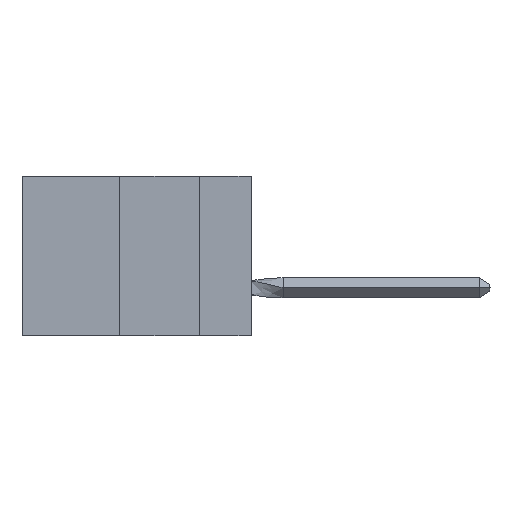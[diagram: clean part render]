
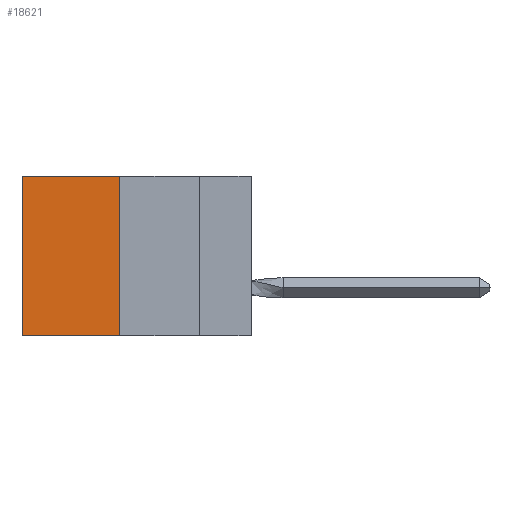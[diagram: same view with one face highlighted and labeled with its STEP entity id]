
A CAD part, left-side view. The second image highlights one B-rep face of the part: STEP entity #18621.
In plain terms, the highlighted planar face has unit normal (-1, 0, 0).
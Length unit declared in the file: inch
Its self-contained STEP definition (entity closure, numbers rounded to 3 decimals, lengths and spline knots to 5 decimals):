
#659 = CARTESIAN_POINT ( 'NONE',  ( 0.305, 0.72, 0. ) ) ;
#1012 = ORIENTED_EDGE ( 'NONE', *, *, #14204, .T. ) ;
#1223 = LINE ( 'NONE', #9986, #7624 ) ;
#3802 = VECTOR ( 'NONE', #15331, 39.37008 ) ;
#3826 = CARTESIAN_POINT ( 'NONE',  ( 0.305, 0.413, -0.5 ) ) ;
#4226 = EDGE_LOOP ( 'NONE', ( #1012, #16216, #18275, #17944 ) ) ;
#4917 = VERTEX_POINT ( 'NONE', #7434 ) ;
#5154 = DIRECTION ( 'NONE',  ( 0., 1., 0. ) ) ;
#5489 = VERTEX_POINT ( 'NONE', #659 ) ;
#5860 = EDGE_CURVE ( 'NONE', #14574, #5489, #9058, .T. ) ;
#5994 = PLANE ( 'NONE',  #16144 ) ;
#6012 = VERTEX_POINT ( 'NONE', #8683 ) ;
#7107 = EDGE_CURVE ( 'NONE', #14574, #6012, #1223, .T. ) ;
#7379 = VECTOR ( 'NONE', #14144, 39.37008 ) ;
#7434 = CARTESIAN_POINT ( 'NONE',  ( 0.305, 0.72, -0.5 ) ) ;
#7554 = DIRECTION ( 'NONE',  ( 1., 0., 0. ) ) ;
#7624 = VECTOR ( 'NONE', #13028, 39.37008 ) ;
#8250 = EDGE_CURVE ( 'NONE', #6012, #4917, #9184, .T. ) ;
#8683 = CARTESIAN_POINT ( 'NONE',  ( 0.305, 0.413, -0.5 ) ) ;
#8724 = VECTOR ( 'NONE', #5154, 39.37008 ) ;
#9058 = LINE ( 'NONE', #13910, #3802 ) ;
#9184 = LINE ( 'NONE', #3826, #8724 ) ;
#9986 = CARTESIAN_POINT ( 'NONE',  ( 0.305, 0.413, -0.5 ) ) ;
#12553 = CARTESIAN_POINT ( 'NONE',  ( 0.305, 0.72, -0.5 ) ) ;
#12854 = LINE ( 'NONE', #12553, #7379 ) ;
#13028 = DIRECTION ( 'NONE',  ( 0., 0., -1. ) ) ;
#13484 = DIRECTION ( 'NONE',  ( 0., 0., -1. ) ) ;
#13910 = CARTESIAN_POINT ( 'NONE',  ( 0.305, 0.413, 0. ) ) ;
#14144 = DIRECTION ( 'NONE',  ( 0., 0., -1. ) ) ;
#14204 = EDGE_CURVE ( 'NONE', #5489, #4917, #12854, .T. ) ;
#14574 = VERTEX_POINT ( 'NONE', #16094 ) ;
#14613 = CARTESIAN_POINT ( 'NONE',  ( 0.305, 0.413, -0.5 ) ) ;
#15331 = DIRECTION ( 'NONE',  ( 0., 1., 0. ) ) ;
#16094 = CARTESIAN_POINT ( 'NONE',  ( 0.305, 0.413, 0. ) ) ;
#16144 = AXIS2_PLACEMENT_3D ( 'NONE', #14613, #7554, #13484 ) ;
#16216 = ORIENTED_EDGE ( 'NONE', *, *, #8250, .F. ) ;
#17944 = ORIENTED_EDGE ( 'NONE', *, *, #5860, .T. ) ;
#18275 = ORIENTED_EDGE ( 'NONE', *, *, #7107, .F. ) ;
#18621 = ADVANCED_FACE ( 'NONE', ( #18757 ), #5994, .F. ) ;
#18757 = FACE_OUTER_BOUND ( 'NONE', #4226, .T. ) ;
